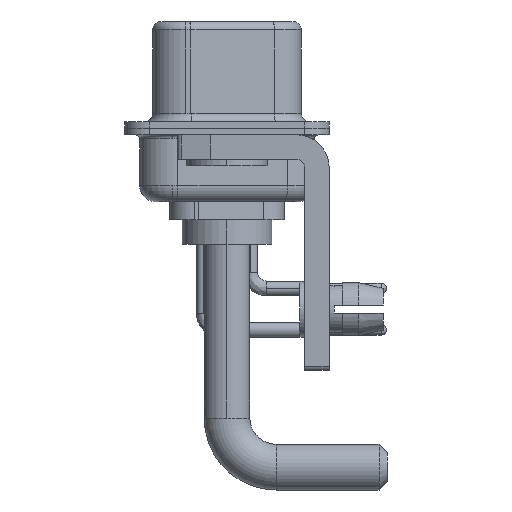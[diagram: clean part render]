
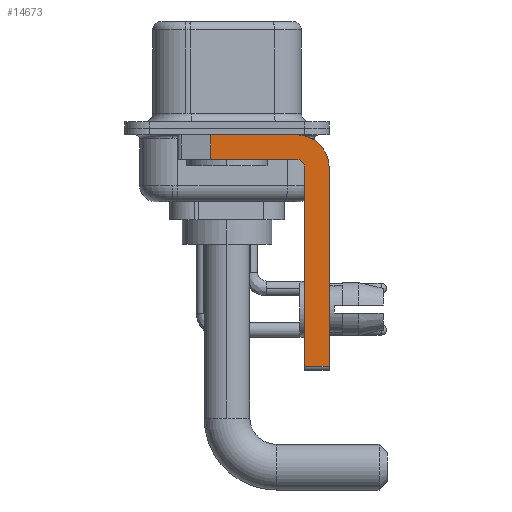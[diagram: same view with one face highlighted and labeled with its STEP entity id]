
A CAD part, left-side view. The second image highlights one B-rep face of the part: STEP entity #14673.
In plain terms, the highlighted planar face has unit normal (-1, 0, 0).
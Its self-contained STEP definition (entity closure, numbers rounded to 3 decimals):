
#366 = CARTESIAN_POINT ( 'NONE',  ( -2.9, -4.25, -1.9 ) ) ;
#1198 = LINE ( 'NONE', #10184, #15901 ) ;
#1762 = DIRECTION ( 'NONE',  ( 0., 0., -1. ) ) ;
#1778 = DIRECTION ( 'NONE',  ( -1., 0., 0. ) ) ;
#2073 = PLANE ( 'NONE',  #6745 ) ;
#2355 = CARTESIAN_POINT ( 'NONE',  ( -2.9, 3., -0.4 ) ) ;
#2370 = ORIENTED_EDGE ( 'NONE', *, *, #3174, .F. ) ;
#3126 = VERTEX_POINT ( 'NONE', #16126 ) ;
#3174 = EDGE_CURVE ( 'NONE', #26481, #26753, #27921, .T. ) ;
#3872 = CARTESIAN_POINT ( 'NONE',  ( -2.9, -6.25, -2.4 ) ) ;
#3880 = CARTESIAN_POINT ( 'NONE',  ( -2.9, -4.25, -14.55 ) ) ;
#4409 = ORIENTED_EDGE ( 'NONE', *, *, #23068, .F. ) ;
#5067 = ORIENTED_EDGE ( 'NONE', *, *, #12748, .F. ) ;
#6165 = CARTESIAN_POINT ( 'NONE',  ( -2.9, -6.25, -2.4 ) ) ;
#6745 = AXIS2_PLACEMENT_3D ( 'NONE', #17408, #24336, #15356 ) ;
#6864 = ORIENTED_EDGE ( 'NONE', *, *, #28274, .F. ) ;
#7196 = ORIENTED_EDGE ( 'NONE', *, *, #12680, .T. ) ;
#7483 = CARTESIAN_POINT ( 'NONE',  ( -2.9, -4.75, -14.55 ) ) ;
#9055 = LINE ( 'NONE', #3880, #23612 ) ;
#9156 = EDGE_CURVE ( 'NONE', #20732, #27632, #9209, .T. ) ;
#9209 = CIRCLE ( 'NONE', #9667, 2. ) ;
#9667 = AXIS2_PLACEMENT_3D ( 'NONE', #26108, #10915, #17397 ) ;
#10184 = CARTESIAN_POINT ( 'NONE',  ( -2.9, 0.978, -1.9 ) ) ;
#10817 = DIRECTION ( 'NONE',  ( 0., -1., 0. ) ) ;
#10915 = DIRECTION ( 'NONE',  ( 1., 0., 0. ) ) ;
#10981 = VERTEX_POINT ( 'NONE', #27202 ) ;
#12548 = DIRECTION ( 'NONE',  ( 0., 0., 1. ) ) ;
#12680 = EDGE_CURVE ( 'NONE', #22281, #26753, #1198, .T. ) ;
#12748 = EDGE_CURVE ( 'NONE', #27632, #3126, #12816, .T. ) ;
#12816 = LINE ( 'NONE', #6165, #25682 ) ;
#13084 = VERTEX_POINT ( 'NONE', #7483 ) ;
#14100 = VECTOR ( 'NONE', #16695, 1000. ) ;
#14595 = LINE ( 'NONE', #25651, #25958 ) ;
#14673 = ADVANCED_FACE ( 'NONE', ( #22119 ), #2073, .F. ) ;
#15356 = DIRECTION ( 'NONE',  ( 0., 0., -1. ) ) ;
#15895 = CARTESIAN_POINT ( 'NONE',  ( -2.9, 0.978, -1.9 ) ) ;
#15901 = VECTOR ( 'NONE', #25797, 1000. ) ;
#16047 = ORIENTED_EDGE ( 'NONE', *, *, #9156, .F. ) ;
#16126 = CARTESIAN_POINT ( 'NONE',  ( -2.9, -6.25, -14.55 ) ) ;
#16695 = DIRECTION ( 'NONE',  ( 0., 1., 0. ) ) ;
#17397 = DIRECTION ( 'NONE',  ( 0., 0., -1. ) ) ;
#17408 = CARTESIAN_POINT ( 'NONE',  ( -2.9, -4.25, -2.4 ) ) ;
#17518 = CARTESIAN_POINT ( 'NONE',  ( -2.9, -4.25, -0.4 ) ) ;
#20205 = EDGE_CURVE ( 'NONE', #10981, #26481, #24189, .T. ) ;
#20632 = DIRECTION ( 'NONE',  ( 0., -1., 0. ) ) ;
#20732 = VERTEX_POINT ( 'NONE', #17518 ) ;
#21856 = ORIENTED_EDGE ( 'NONE', *, *, #28684, .T. ) ;
#21967 = CARTESIAN_POINT ( 'NONE',  ( -2.9, -4.25, -2.4 ) ) ;
#22108 = ORIENTED_EDGE ( 'NONE', *, *, #20205, .F. ) ;
#22119 = FACE_OUTER_BOUND ( 'NONE', #27670, .T. ) ;
#22281 = VERTEX_POINT ( 'NONE', #25998 ) ;
#22318 = AXIS2_PLACEMENT_3D ( 'NONE', #21967, #1778, #12548 ) ;
#22441 = CARTESIAN_POINT ( 'NONE',  ( -2.9, -4.25, -1.9 ) ) ;
#22699 = LINE ( 'NONE', #2355, #28521 ) ;
#23068 = EDGE_CURVE ( 'NONE', #22281, #20732, #22699, .T. ) ;
#23286 = DIRECTION ( 'NONE',  ( 0., 0., 1. ) ) ;
#23612 = VECTOR ( 'NONE', #10817, 1000. ) ;
#24189 = CIRCLE ( 'NONE', #22318, 0.5 ) ;
#24336 = DIRECTION ( 'NONE',  ( 1., 0., 0. ) ) ;
#25651 = CARTESIAN_POINT ( 'NONE',  ( -2.9, -4.75, -14.8 ) ) ;
#25682 = VECTOR ( 'NONE', #1762, 1000. ) ;
#25797 = DIRECTION ( 'NONE',  ( 0., 0., -1. ) ) ;
#25958 = VECTOR ( 'NONE', #23286, 1000. ) ;
#25998 = CARTESIAN_POINT ( 'NONE',  ( -2.9, 0.978, -0.4 ) ) ;
#26108 = CARTESIAN_POINT ( 'NONE',  ( -2.9, -4.25, -2.4 ) ) ;
#26481 = VERTEX_POINT ( 'NONE', #22441 ) ;
#26753 = VERTEX_POINT ( 'NONE', #15895 ) ;
#27202 = CARTESIAN_POINT ( 'NONE',  ( -2.9, -4.75, -2.4 ) ) ;
#27632 = VERTEX_POINT ( 'NONE', #3872 ) ;
#27670 = EDGE_LOOP ( 'NONE', ( #4409, #7196, #2370, #22108, #6864, #21856, #5067, #16047 ) ) ;
#27921 = LINE ( 'NONE', #366, #14100 ) ;
#28274 = EDGE_CURVE ( 'NONE', #13084, #10981, #14595, .T. ) ;
#28521 = VECTOR ( 'NONE', #20632, 1000. ) ;
#28684 = EDGE_CURVE ( 'NONE', #13084, #3126, #9055, .T. ) ;
